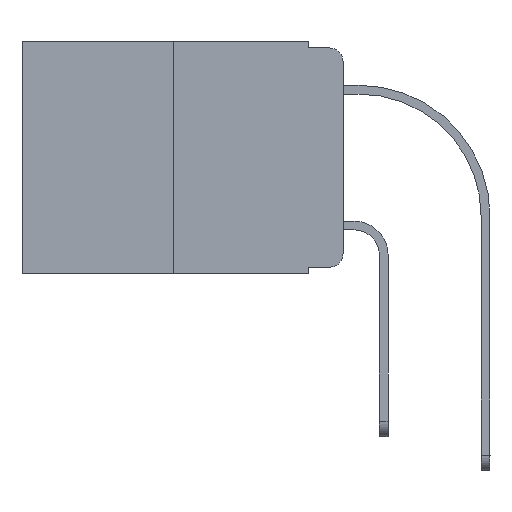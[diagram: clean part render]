
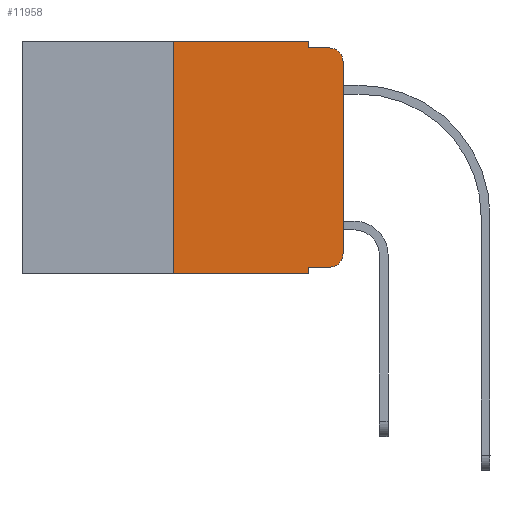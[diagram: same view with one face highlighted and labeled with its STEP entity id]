
A CAD part, left-side view. The second image highlights one B-rep face of the part: STEP entity #11958.
In plain terms, the highlighted planar face has unit normal (-1, 0, 0).
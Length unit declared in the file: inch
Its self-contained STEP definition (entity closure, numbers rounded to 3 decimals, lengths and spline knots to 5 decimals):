
#148 = CARTESIAN_POINT ( 'NONE',  ( 0., 0.02, -0.03 ) ) ;
#290 = ORIENTED_EDGE ( 'NONE', *, *, #19791, .F. ) ;
#302 = AXIS2_PLACEMENT_3D ( 'NONE', #21222, #20766, #3283 ) ;
#303 = LINE ( 'NONE', #21249, #10634 ) ;
#347 = ORIENTED_EDGE ( 'NONE', *, *, #1662, .T. ) ;
#1015 = ORIENTED_EDGE ( 'NONE', *, *, #12928, .F. ) ;
#1662 = EDGE_CURVE ( 'NONE', #14876, #19540, #5998, .T. ) ;
#1699 = EDGE_CURVE ( 'NONE', #18257, #14876, #15196, .T. ) ;
#1995 = DIRECTION ( 'NONE',  ( 0., 0., -1. ) ) ;
#2875 = EDGE_CURVE ( 'NONE', #15583, #14617, #15700, .T. ) ;
#2994 = ORIENTED_EDGE ( 'NONE', *, *, #2875, .T. ) ;
#3283 = DIRECTION ( 'NONE',  ( 0., 0., -1. ) ) ;
#3336 = LINE ( 'NONE', #4945, #8943 ) ;
#3382 = CARTESIAN_POINT ( 'NONE',  ( 0., 0.473, -0.343 ) ) ;
#3795 = DIRECTION ( 'NONE',  ( 0., -1., 0. ) ) ;
#3958 = CARTESIAN_POINT ( 'NONE',  ( 0., 0.25, 0. ) ) ;
#4394 = CARTESIAN_POINT ( 'NONE',  ( 0., 0.25, -0.343 ) ) ;
#4547 = VECTOR ( 'NONE', #5937, 39.37008 ) ;
#4945 = CARTESIAN_POINT ( 'NONE',  ( 0., 0.051, 0. ) ) ;
#5065 = DIRECTION ( 'NONE',  ( 0., 0., -1. ) ) ;
#5930 = CIRCLE ( 'NONE', #10373, 0.02 ) ;
#5937 = DIRECTION ( 'NONE',  ( 0., 0., -1. ) ) ;
#5963 = LINE ( 'NONE', #9436, #17431 ) ;
#5998 = CIRCLE ( 'NONE', #16303, 0.02 ) ;
#6369 = CARTESIAN_POINT ( 'NONE',  ( 0., 0.051, -0.01 ) ) ;
#6376 = ORIENTED_EDGE ( 'NONE', *, *, #1699, .T. ) ;
#6569 = EDGE_CURVE ( 'NONE', #22183, #11617, #3336, .T. ) ;
#6736 = VECTOR ( 'NONE', #3795, 39.37008 ) ;
#6759 = DIRECTION ( 'NONE',  ( 0., 0., -1. ) ) ;
#7551 = DIRECTION ( 'NONE',  ( 0., -1., 0. ) ) ;
#8180 = EDGE_CURVE ( 'NONE', #13743, #18257, #5930, .T. ) ;
#8610 = DIRECTION ( 'NONE',  ( -1., 0., 0. ) ) ;
#8797 = DIRECTION ( 'NONE',  ( -1., 0., 0. ) ) ;
#8943 = VECTOR ( 'NONE', #5065, 39.37008 ) ;
#9011 = CARTESIAN_POINT ( 'NONE',  ( 0., 0.02, -0.333 ) ) ;
#9137 = DIRECTION ( 'NONE',  ( 0., -1., 0. ) ) ;
#9349 = ORIENTED_EDGE ( 'NONE', *, *, #16426, .F. ) ;
#9436 = CARTESIAN_POINT ( 'NONE',  ( 0., 0.25, 0. ) ) ;
#10373 = AXIS2_PLACEMENT_3D ( 'NONE', #20791, #8610, #6759 ) ;
#10634 = VECTOR ( 'NONE', #7551, 39.37008 ) ;
#11617 = VERTEX_POINT ( 'NONE', #6369 ) ;
#11839 = ORIENTED_EDGE ( 'NONE', *, *, #6569, .F. ) ;
#11958 = ADVANCED_FACE ( 'NONE', ( #12041 ), #15709, .F. ) ;
#12041 = FACE_OUTER_BOUND ( 'NONE', #12339, .T. ) ;
#12339 = EDGE_LOOP ( 'NONE', ( #6376, #347, #1015, #11839, #9349, #290, #2994, #22216, #17004, #13576 ) ) ;
#12928 = EDGE_CURVE ( 'NONE', #11617, #19540, #17716, .T. ) ;
#13576 = ORIENTED_EDGE ( 'NONE', *, *, #8180, .T. ) ;
#13743 = VERTEX_POINT ( 'NONE', #9011 ) ;
#14617 = VERTEX_POINT ( 'NONE', #16302 ) ;
#14668 = CARTESIAN_POINT ( 'NONE',  ( 0., 0.02, -0.01 ) ) ;
#14697 = CARTESIAN_POINT ( 'NONE',  ( 0., 0.051, 0. ) ) ;
#14781 = EDGE_CURVE ( 'NONE', #20555, #14617, #18134, .T. ) ;
#14876 = VERTEX_POINT ( 'NONE', #17207 ) ;
#15196 = LINE ( 'NONE', #22429, #19708 ) ;
#15583 = VERTEX_POINT ( 'NONE', #4394 ) ;
#15700 = LINE ( 'NONE', #3382, #21516 ) ;
#15709 = PLANE ( 'NONE',  #302 ) ;
#16302 = CARTESIAN_POINT ( 'NONE',  ( 0., 0.051, -0.343 ) ) ;
#16303 = AXIS2_PLACEMENT_3D ( 'NONE', #148, #8797, #1995 ) ;
#16426 = EDGE_CURVE ( 'NONE', #19380, #22183, #18085, .T. ) ;
#16437 = DIRECTION ( 'NONE',  ( 0., 0., 1. ) ) ;
#16955 = DIRECTION ( 'NONE',  ( 0., -1., 0. ) ) ;
#17004 = ORIENTED_EDGE ( 'NONE', *, *, #17758, .T. ) ;
#17021 = CARTESIAN_POINT ( 'NONE',  ( 0., 0., -0.313 ) ) ;
#17207 = CARTESIAN_POINT ( 'NONE',  ( 0., 0., -0.03 ) ) ;
#17431 = VECTOR ( 'NONE', #16437, 39.37008 ) ;
#17716 = LINE ( 'NONE', #19338, #6736 ) ;
#17758 = EDGE_CURVE ( 'NONE', #20555, #13743, #303, .T. ) ;
#18085 = LINE ( 'NONE', #19928, #18701 ) ;
#18134 = LINE ( 'NONE', #14697, #4547 ) ;
#18257 = VERTEX_POINT ( 'NONE', #17021 ) ;
#18557 = CARTESIAN_POINT ( 'NONE',  ( 0., 0.051, 0. ) ) ;
#18701 = VECTOR ( 'NONE', #9137, 39.37008 ) ;
#19338 = CARTESIAN_POINT ( 'NONE',  ( 0., 0.051, -0.01 ) ) ;
#19380 = VERTEX_POINT ( 'NONE', #3958 ) ;
#19540 = VERTEX_POINT ( 'NONE', #14668 ) ;
#19708 = VECTOR ( 'NONE', #22201, 39.37008 ) ;
#19791 = EDGE_CURVE ( 'NONE', #15583, #19380, #5963, .T. ) ;
#19928 = CARTESIAN_POINT ( 'NONE',  ( 0., 0.473, 0. ) ) ;
#20555 = VERTEX_POINT ( 'NONE', #22473 ) ;
#20766 = DIRECTION ( 'NONE',  ( 1., 0., 0. ) ) ;
#20791 = CARTESIAN_POINT ( 'NONE',  ( 0., 0.02, -0.313 ) ) ;
#21222 = CARTESIAN_POINT ( 'NONE',  ( 0., 0.473, 0. ) ) ;
#21249 = CARTESIAN_POINT ( 'NONE',  ( 0., 0.051, -0.333 ) ) ;
#21516 = VECTOR ( 'NONE', #16955, 39.37008 ) ;
#22183 = VERTEX_POINT ( 'NONE', #18557 ) ;
#22201 = DIRECTION ( 'NONE',  ( 0., 0., 1. ) ) ;
#22216 = ORIENTED_EDGE ( 'NONE', *, *, #14781, .F. ) ;
#22429 = CARTESIAN_POINT ( 'NONE',  ( 0., 0., 0. ) ) ;
#22473 = CARTESIAN_POINT ( 'NONE',  ( 0., 0.051, -0.333 ) ) ;
